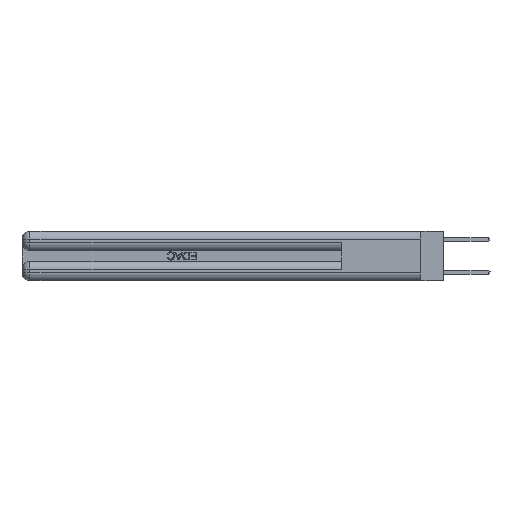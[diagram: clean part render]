
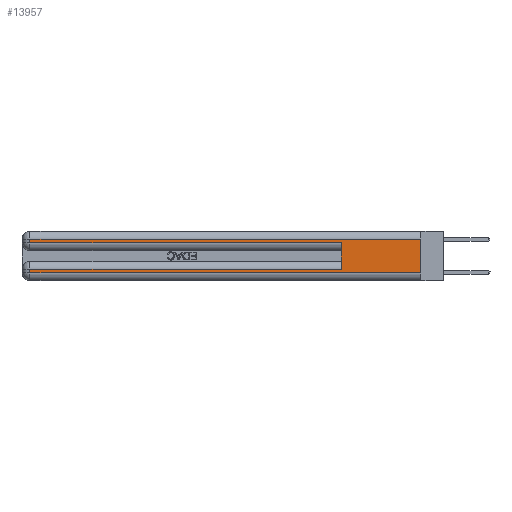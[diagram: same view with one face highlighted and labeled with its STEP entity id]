
A CAD part, left-side view. The second image highlights one B-rep face of the part: STEP entity #13957.
In plain terms, the highlighted planar face has unit normal (-1, 0, 0).
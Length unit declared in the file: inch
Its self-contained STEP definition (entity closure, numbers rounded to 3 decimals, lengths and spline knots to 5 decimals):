
#1269 = PLANE ( 'NONE',  #12530 ) ;
#1640 = CARTESIAN_POINT ( 'NONE',  ( 0., 0., 0.285 ) ) ;
#1966 = LINE ( 'NONE', #25749, #24413 ) ;
#2024 = VECTOR ( 'NONE', #27702, 39.37008 ) ;
#2136 = CARTESIAN_POINT ( 'NONE',  ( 0., 0., 0.06 ) ) ;
#3020 = EDGE_CURVE ( 'NONE', #25623, #9475, #11932, .T. ) ;
#3122 = ORIENTED_EDGE ( 'NONE', *, *, #9918, .T. ) ;
#3132 = CARTESIAN_POINT ( 'NONE',  ( 0., 0.6, 0.285 ) ) ;
#3675 = VERTEX_POINT ( 'NONE', #2136 ) ;
#3695 = VECTOR ( 'NONE', #8323, 39.37008 ) ;
#3978 = ORIENTED_EDGE ( 'NONE', *, *, #27884, .T. ) ;
#5074 = DIRECTION ( 'NONE',  ( 0., -1., 0. ) ) ;
#5672 = DIRECTION ( 'NONE',  ( 1., 0., 0. ) ) ;
#6048 = DIRECTION ( 'NONE',  ( 0., -1., 0. ) ) ;
#6137 = VECTOR ( 'NONE', #12972, 39.37008 ) ;
#7266 = VECTOR ( 'NONE', #6048, 39.37008 ) ;
#7963 = LINE ( 'NONE', #1640, #7266 ) ;
#8013 = CARTESIAN_POINT ( 'NONE',  ( 0., 0., 0.085 ) ) ;
#8323 = DIRECTION ( 'NONE',  ( 0., 0., 1. ) ) ;
#8330 = LINE ( 'NONE', #15696, #24899 ) ;
#9475 = VERTEX_POINT ( 'NONE', #13353 ) ;
#9542 = LINE ( 'NONE', #10406, #3695 ) ;
#9770 = CARTESIAN_POINT ( 'NONE',  ( 0., 0., 0.31 ) ) ;
#9918 = EDGE_CURVE ( 'NONE', #11312, #12209, #21604, .T. ) ;
#10406 = CARTESIAN_POINT ( 'NONE',  ( 0., 0.6, 0.145 ) ) ;
#10528 = ORIENTED_EDGE ( 'NONE', *, *, #27605, .T. ) ;
#10652 = EDGE_CURVE ( 'NONE', #12209, #10691, #8330, .T. ) ;
#10691 = VERTEX_POINT ( 'NONE', #22321 ) ;
#10952 = EDGE_CURVE ( 'NONE', #23761, #20621, #7963, .T. ) ;
#11312 = VERTEX_POINT ( 'NONE', #14043 ) ;
#11932 = LINE ( 'NONE', #23758, #6137 ) ;
#12209 = VERTEX_POINT ( 'NONE', #27599 ) ;
#12530 = AXIS2_PLACEMENT_3D ( 'NONE', #18735, #5672, #20910 ) ;
#12972 = DIRECTION ( 'NONE',  ( 0., 1., 0. ) ) ;
#13353 = CARTESIAN_POINT ( 'NONE',  ( 0., 2.94, 0.31 ) ) ;
#13647 = LINE ( 'NONE', #21226, #2024 ) ;
#13957 = ADVANCED_FACE ( 'NONE', ( #26747 ), #1269, .F. ) ;
#14043 = CARTESIAN_POINT ( 'NONE',  ( 0., 0.6, 0.085 ) ) ;
#15181 = VECTOR ( 'NONE', #21033, 39.37008 ) ;
#15696 = CARTESIAN_POINT ( 'NONE',  ( 0., 2.94, 0.37 ) ) ;
#15942 = CARTESIAN_POINT ( 'NONE',  ( 0., 0., 0.06 ) ) ;
#16980 = VECTOR ( 'NONE', #5074, 39.37008 ) ;
#17204 = DIRECTION ( 'NONE',  ( 0., 0., -1. ) ) ;
#17874 = DIRECTION ( 'NONE',  ( 0., 0., -1. ) ) ;
#18101 = ORIENTED_EDGE ( 'NONE', *, *, #10652, .T. ) ;
#18358 = EDGE_CURVE ( 'NONE', #25623, #3675, #13647, .T. ) ;
#18538 = CARTESIAN_POINT ( 'NONE',  ( 0., 2.94, 0.285 ) ) ;
#18735 = CARTESIAN_POINT ( 'NONE',  ( 0., 0., 0.37 ) ) ;
#18990 = EDGE_CURVE ( 'NONE', #11312, #20621, #9542, .T. ) ;
#19211 = EDGE_LOOP ( 'NONE', ( #24878, #24020, #10528, #20003, #22525, #3122, #18101, #3978 ) ) ;
#20003 = ORIENTED_EDGE ( 'NONE', *, *, #10952, .T. ) ;
#20621 = VERTEX_POINT ( 'NONE', #3132 ) ;
#20910 = DIRECTION ( 'NONE',  ( 0., 0., -1. ) ) ;
#21033 = DIRECTION ( 'NONE',  ( 0., 1., 0. ) ) ;
#21226 = CARTESIAN_POINT ( 'NONE',  ( 0., 0., 0.37 ) ) ;
#21604 = LINE ( 'NONE', #8013, #15181 ) ;
#22321 = CARTESIAN_POINT ( 'NONE',  ( 0., 2.94, 0.06 ) ) ;
#22525 = ORIENTED_EDGE ( 'NONE', *, *, #18990, .F. ) ;
#22719 = LINE ( 'NONE', #15942, #16980 ) ;
#23758 = CARTESIAN_POINT ( 'NONE',  ( 0., 0., 0.31 ) ) ;
#23761 = VERTEX_POINT ( 'NONE', #18538 ) ;
#24020 = ORIENTED_EDGE ( 'NONE', *, *, #3020, .T. ) ;
#24413 = VECTOR ( 'NONE', #17204, 39.37008 ) ;
#24878 = ORIENTED_EDGE ( 'NONE', *, *, #18358, .F. ) ;
#24899 = VECTOR ( 'NONE', #17874, 39.37008 ) ;
#25623 = VERTEX_POINT ( 'NONE', #9770 ) ;
#25749 = CARTESIAN_POINT ( 'NONE',  ( 0., 2.94, 0.37 ) ) ;
#26747 = FACE_OUTER_BOUND ( 'NONE', #19211, .T. ) ;
#27599 = CARTESIAN_POINT ( 'NONE',  ( 0., 2.94, 0.085 ) ) ;
#27605 = EDGE_CURVE ( 'NONE', #9475, #23761, #1966, .T. ) ;
#27702 = DIRECTION ( 'NONE',  ( 0., 0., -1. ) ) ;
#27884 = EDGE_CURVE ( 'NONE', #10691, #3675, #22719, .T. ) ;
